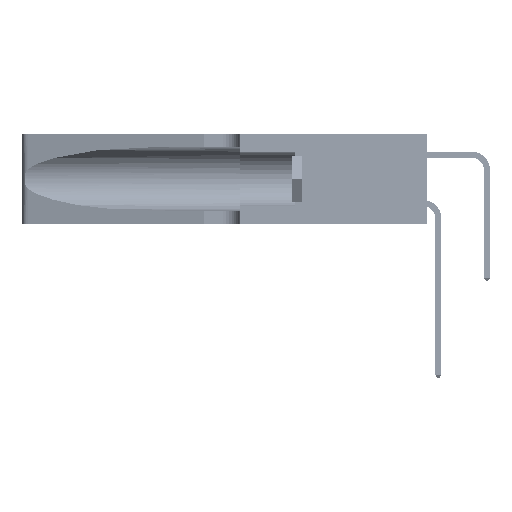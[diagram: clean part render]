
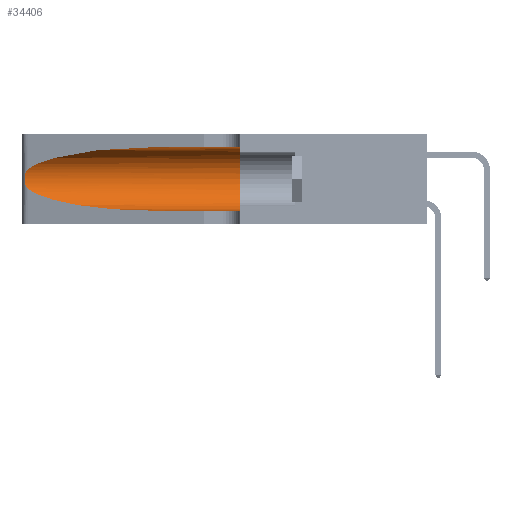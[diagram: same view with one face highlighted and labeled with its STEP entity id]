
A CAD part, left-side view. The second image highlights one B-rep face of the part: STEP entity #34406.
In plain terms, the highlighted cylindrical face has radius 3.308 mm (diameter 6.617 mm), a partial arc.
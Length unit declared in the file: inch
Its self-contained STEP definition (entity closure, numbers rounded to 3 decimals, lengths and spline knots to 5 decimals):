
#209 = DIRECTION ( 'NONE',  ( 0., 0., -1. ) ) ;
#2675 = CARTESIAN_POINT ( 'NONE',  ( 0.26075, 1.23896, 0.178 ) ) ;
#3424 = VERTEX_POINT ( 'NONE', #38548 ) ;
#3892 = DIRECTION ( 'NONE',  ( 0., -1., 0. ) ) ;
#5978 = CARTESIAN_POINT ( 'NONE',  ( 0.25487, 1.22718, 0.22369 ) ) ;
#6641 = CARTESIAN_POINT ( 'NONE',  ( 0.25856, 1.23593, 0.16098 ) ) ;
#6952 = VERTEX_POINT ( 'NONE', #43472 ) ;
#9391 = VECTOR ( 'NONE', #3892, 39.37008 ) ;
#10447 = CARTESIAN_POINT ( 'NONE',  ( 0.25555, 1.22994, 0.2215 ) ) ;
#10619 = CARTESIAN_POINT ( 'NONE',  ( 0.25639, 1.23186, 0.15144 ) ) ;
#12189 = EDGE_CURVE ( 'NONE', #13342, #20813, #28901, .T. ) ;
#12614 = CARTESIAN_POINT ( 'NONE',  ( 0.1305, 0.35, 0.185 ) ) ;
#13342 = VERTEX_POINT ( 'NONE', #16128 ) ;
#14576 = CARTESIAN_POINT ( 'NONE',  ( 0.25487, 1.22718, 0.14631 ) ) ;
#14675 =( BOUNDED_CURVE ( )  B_SPLINE_CURVE ( 3, ( #44921, #33180, #29404, #5978 ),
 .UNSPECIFIED., .F., .F. ) 
 B_SPLINE_CURVE_WITH_KNOTS ( ( 4, 4 ),
 ( 1.5708, 2.84003 ),
 .UNSPECIFIED. ) 
 CURVE ( )  GEOMETRIC_REPRESENTATION_ITEM ( )  RATIONAL_B_SPLINE_CURVE ( ( 1., 0.87, 0.87, 1. ) ) 
 REPRESENTATION_ITEM ( '' )  );
#14916 = EDGE_CURVE ( 'NONE', #13342, #3424, #14675, .T. ) ;
#15029 = EDGE_CURVE ( 'NONE', #28845, #6952, #33600, .T. ) ;
#15523 = CARTESIAN_POINT ( 'NONE',  ( 0.2373, 1.15595, 0.08982 ) ) ;
#16128 = CARTESIAN_POINT ( 'NONE',  ( 0.1305, 0.72297, 0.31525 ) ) ;
#16541 = DIRECTION ( 'NONE',  ( 0., 0., 1. ) ) ;
#16744 = VERTEX_POINT ( 'NONE', #28095 ) ;
#18316 = CARTESIAN_POINT ( 'NONE',  ( 0.25639, 1.23184, 0.21858 ) ) ;
#20813 = VERTEX_POINT ( 'NONE', #35452 ) ;
#21111 = CIRCLE ( 'NONE', #49551, 0.13025 ) ;
#21993 = VECTOR ( 'NONE', #37774, 39.37008 ) ;
#22209 = CARTESIAN_POINT ( 'NONE',  ( 0.25854, 1.2359, 0.20912 ) ) ;
#23390 = CARTESIAN_POINT ( 'NONE',  ( 0.1305, 1.61858, 0.31525 ) ) ;
#25712 = EDGE_LOOP ( 'NONE', ( #37898, #35131, #42034, #42363, #35932, #47334 ) ) ;
#26108 = CARTESIAN_POINT ( 'NONE',  ( 0.26075, 1.23896, 0.19203 ) ) ;
#27234 = CARTESIAN_POINT ( 'NONE',  ( 0.1305, 0.72297, 0.05475 ) ) ;
#28095 = CARTESIAN_POINT ( 'NONE',  ( 0.25487, 1.22718, 0.14631 ) ) ;
#28155 = EDGE_CURVE ( 'NONE', #16744, #28845, #38079, .T. ) ;
#28845 = VERTEX_POINT ( 'NONE', #31787 ) ;
#28901 = LINE ( 'NONE', #23390, #9391 ) ;
#29404 = CARTESIAN_POINT ( 'NONE',  ( 0.2373, 1.15595, 0.28018 ) ) ;
#30030 = CARTESIAN_POINT ( 'NONE',  ( 0.26017, 1.23833, 0.17102 ) ) ;
#30935 = AXIS2_PLACEMENT_3D ( 'NONE', #43110, #35306, #209 ) ;
#31787 = CARTESIAN_POINT ( 'NONE',  ( 0.1305, 0.72297, 0.05475 ) ) ;
#33180 = CARTESIAN_POINT ( 'NONE',  ( 0.18966, 0.96281, 0.31525 ) ) ;
#33600 = LINE ( 'NONE', #45584, #21993 ) ;
#33979 = CARTESIAN_POINT ( 'NONE',  ( 0.25789, 1.23486, 0.15765 ) ) ;
#34406 = ADVANCED_FACE ( 'NONE', ( #41286 ), #40075, .F. ) ;
#35131 = ORIENTED_EDGE ( 'NONE', *, *, #46563, .T. ) ;
#35306 = DIRECTION ( 'NONE',  ( 0., -1., 0. ) ) ;
#35452 = CARTESIAN_POINT ( 'NONE',  ( 0.1305, 0.35, 0.31525 ) ) ;
#35932 = ORIENTED_EDGE ( 'NONE', *, *, #36488, .F. ) ;
#36488 = EDGE_CURVE ( 'NONE', #20813, #6952, #21111, .T. ) ;
#37741 = CARTESIAN_POINT ( 'NONE',  ( 0.25487, 1.22718, 0.22369 ) ) ;
#37774 = DIRECTION ( 'NONE',  ( 0., -1., 0. ) ) ;
#37898 = ORIENTED_EDGE ( 'NONE', *, *, #14916, .T. ) ;
#37902 = CARTESIAN_POINT ( 'NONE',  ( 0.25555, 1.22993, 0.14849 ) ) ;
#38079 =( BOUNDED_CURVE ( )  B_SPLINE_CURVE ( 3, ( #46663, #15523, #50557, #27234 ),
 .UNSPECIFIED., .F., .F. ) 
 B_SPLINE_CURVE_WITH_KNOTS ( ( 4, 4 ),
 ( 3.44316, 4.71239 ),
 .UNSPECIFIED. ) 
 CURVE ( )  GEOMETRIC_REPRESENTATION_ITEM ( )  RATIONAL_B_SPLINE_CURVE ( ( 1., 0.87, 0.87, 1. ) ) 
 REPRESENTATION_ITEM ( '' )  );
#38548 = CARTESIAN_POINT ( 'NONE',  ( 0.25487, 1.22718, 0.22369 ) ) ;
#39836 = DIRECTION ( 'NONE',  ( 0., 1., 0. ) ) ;
#40075 = CYLINDRICAL_SURFACE ( 'NONE', #30935, 0.13025 ) ;
#41286 = FACE_OUTER_BOUND ( 'NONE', #25712, .T. ) ;
#42034 = ORIENTED_EDGE ( 'NONE', *, *, #28155, .T. ) ;
#42363 = ORIENTED_EDGE ( 'NONE', *, *, #15029, .T. ) ;
#43110 = CARTESIAN_POINT ( 'NONE',  ( 0.1305, 1.61858, 0.185 ) ) ;
#43472 = CARTESIAN_POINT ( 'NONE',  ( 0.1305, 0.35, 0.05475 ) ) ;
#44921 = CARTESIAN_POINT ( 'NONE',  ( 0.1305, 0.72297, 0.31525 ) ) ;
#45547 = CARTESIAN_POINT ( 'NONE',  ( 0.25787, 1.23484, 0.2124 ) ) ;
#45584 = CARTESIAN_POINT ( 'NONE',  ( 0.1305, 1.61858, 0.05475 ) ) ;
#46563 = EDGE_CURVE ( 'NONE', #3424, #16744, #48656, .T. ) ;
#46663 = CARTESIAN_POINT ( 'NONE',  ( 0.25487, 1.22718, 0.14631 ) ) ;
#47334 = ORIENTED_EDGE ( 'NONE', *, *, #12189, .F. ) ;
#48656 = B_SPLINE_CURVE_WITH_KNOTS ( 'NONE', 3,
 ( #37741, #10447, #18316, #45547, #22209, #49427, #26108, #2675, #30030, #6641, #33979, #10619, #37902, #14576 ),
 .UNSPECIFIED., .F., .F.,
 ( 4, 2, 2, 2, 2, 2, 4 ),
 ( 0., 0.00027, 0.00053, 0.00107, 0.0016, 0.00187, 0.00214 ),
 .UNSPECIFIED. ) ;
#49427 = CARTESIAN_POINT ( 'NONE',  ( 0.26018, 1.23835, 0.19895 ) ) ;
#49551 = AXIS2_PLACEMENT_3D ( 'NONE', #12614, #39836, #16541 ) ;
#50557 = CARTESIAN_POINT ( 'NONE',  ( 0.18966, 0.96281, 0.05475 ) ) ;
